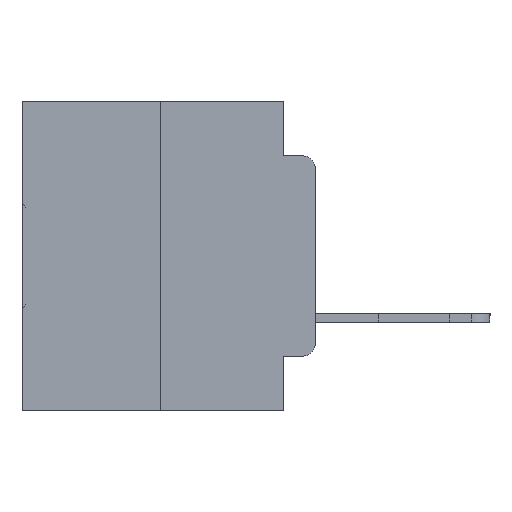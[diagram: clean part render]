
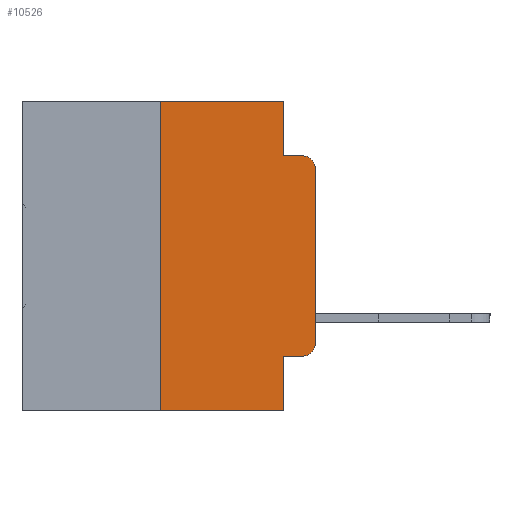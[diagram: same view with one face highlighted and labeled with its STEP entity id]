
A CAD part, left-side view. The second image highlights one B-rep face of the part: STEP entity #10526.
In plain terms, the highlighted planar face has unit normal (-1, 0, 0).
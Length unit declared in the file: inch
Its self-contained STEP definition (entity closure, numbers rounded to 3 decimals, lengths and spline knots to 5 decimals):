
#678 = DIRECTION ( 'NONE',  ( 0., 0., -1. ) ) ;
#717 = DIRECTION ( 'NONE',  ( 0., 0., -1. ) ) ;
#792 = LINE ( 'NONE', #27211, #8308 ) ;
#1229 = DIRECTION ( 'NONE',  ( 0., 0., -1. ) ) ;
#1414 = DIRECTION ( 'NONE',  ( 0., -1., 0. ) ) ;
#2247 = CARTESIAN_POINT ( 'NONE',  ( 0., 0.051, -0.4115 ) ) ;
#2288 = EDGE_CURVE ( 'NONE', #13686, #7421, #14480, .T. ) ;
#2513 = CARTESIAN_POINT ( 'NONE',  ( 0., 0.051, -0.4115 ) ) ;
#2768 = VECTOR ( 'NONE', #20639, 39.37008 ) ;
#4235 = VERTEX_POINT ( 'NONE', #22515 ) ;
#4680 = DIRECTION ( 'NONE',  ( 0., 0., 1. ) ) ;
#5183 = VECTOR ( 'NONE', #1414, 39.37008 ) ;
#5195 = LINE ( 'NONE', #11602, #23070 ) ;
#6860 = EDGE_CURVE ( 'NONE', #8019, #24283, #24549, .T. ) ;
#7421 = VERTEX_POINT ( 'NONE', #30618 ) ;
#7901 = CARTESIAN_POINT ( 'NONE',  ( 0., 0., -0.3915 ) ) ;
#8019 = VERTEX_POINT ( 'NONE', #9274 ) ;
#8308 = VECTOR ( 'NONE', #15422, 39.37008 ) ;
#8387 = VERTEX_POINT ( 'NONE', #8701 ) ;
#8701 = CARTESIAN_POINT ( 'NONE',  ( 0., 0.051, -0.0885 ) ) ;
#8848 = EDGE_CURVE ( 'NONE', #7421, #15583, #22178, .T. ) ;
#9274 = CARTESIAN_POINT ( 'NONE',  ( 0., 0.25, -0.5 ) ) ;
#10526 = ADVANCED_FACE ( 'NONE', ( #15390 ), #11221, .F. ) ;
#10783 = CARTESIAN_POINT ( 'NONE',  ( 0., 0.051, -0.5 ) ) ;
#11136 = LINE ( 'NONE', #28332, #27899 ) ;
#11221 = PLANE ( 'NONE',  #29404 ) ;
#11495 = DIRECTION ( 'NONE',  ( 0., 0., -1. ) ) ;
#11602 = CARTESIAN_POINT ( 'NONE',  ( 0., 0.051, 0. ) ) ;
#11718 = DIRECTION ( 'NONE',  ( 0., -1., 0. ) ) ;
#11909 = DIRECTION ( 'NONE',  ( 0., 0., 1. ) ) ;
#11914 = EDGE_CURVE ( 'NONE', #18131, #8387, #5195, .T. ) ;
#12197 = EDGE_CURVE ( 'NONE', #17667, #24283, #792, .T. ) ;
#13686 = VERTEX_POINT ( 'NONE', #7901 ) ;
#13845 = ORIENTED_EDGE ( 'NONE', *, *, #2288, .T. ) ;
#14002 = CARTESIAN_POINT ( 'NONE',  ( 0., 0.051, 0. ) ) ;
#14480 = LINE ( 'NONE', #18011, #27082 ) ;
#14961 = ORIENTED_EDGE ( 'NONE', *, *, #15974, .F. ) ;
#15008 = DIRECTION ( 'NONE',  ( 0., -1., 0. ) ) ;
#15287 = ORIENTED_EDGE ( 'NONE', *, *, #18986, .F. ) ;
#15313 = AXIS2_PLACEMENT_3D ( 'NONE', #29718, #15635, #717 ) ;
#15390 = FACE_OUTER_BOUND ( 'NONE', #15588, .T. ) ;
#15422 = DIRECTION ( 'NONE',  ( 0., 0., -1. ) ) ;
#15583 = VERTEX_POINT ( 'NONE', #19943 ) ;
#15586 = DIRECTION ( 'NONE',  ( -1., 0., 0. ) ) ;
#15588 = EDGE_LOOP ( 'NONE', ( #13845, #24162, #14961, #22343, #17452, #15287, #20679, #16308, #16558, #19122 ) ) ;
#15635 = DIRECTION ( 'NONE',  ( -1., 0., 0. ) ) ;
#15974 = EDGE_CURVE ( 'NONE', #8387, #15583, #11136, .T. ) ;
#16094 = DIRECTION ( 'NONE',  ( 1., 0., 0. ) ) ;
#16308 = ORIENTED_EDGE ( 'NONE', *, *, #12197, .F. ) ;
#16558 = ORIENTED_EDGE ( 'NONE', *, *, #20662, .T. ) ;
#16653 = CARTESIAN_POINT ( 'NONE',  ( 0., 0.25, 0. ) ) ;
#17452 = ORIENTED_EDGE ( 'NONE', *, *, #26345, .F. ) ;
#17667 = VERTEX_POINT ( 'NONE', #2247 ) ;
#18011 = CARTESIAN_POINT ( 'NONE',  ( 0., 0., 0. ) ) ;
#18090 = LINE ( 'NONE', #16653, #23728 ) ;
#18131 = VERTEX_POINT ( 'NONE', #14002 ) ;
#18177 = CARTESIAN_POINT ( 'NONE',  ( 0., 0.473, 0. ) ) ;
#18642 = CARTESIAN_POINT ( 'NONE',  ( 0., 0.473, -0.5 ) ) ;
#18830 = VERTEX_POINT ( 'NONE', #25703 ) ;
#18986 = EDGE_CURVE ( 'NONE', #8019, #4235, #18090, .T. ) ;
#19122 = ORIENTED_EDGE ( 'NONE', *, *, #28321, .T. ) ;
#19943 = CARTESIAN_POINT ( 'NONE',  ( 0., 0.02, -0.0885 ) ) ;
#20639 = DIRECTION ( 'NONE',  ( 0., -1., 0. ) ) ;
#20662 = EDGE_CURVE ( 'NONE', #17667, #18830, #27985, .T. ) ;
#20679 = ORIENTED_EDGE ( 'NONE', *, *, #6860, .T. ) ;
#21016 = VECTOR ( 'NONE', #15008, 39.37008 ) ;
#22178 = CIRCLE ( 'NONE', #27222, 0.02 ) ;
#22285 = LINE ( 'NONE', #18177, #2768 ) ;
#22343 = ORIENTED_EDGE ( 'NONE', *, *, #11914, .F. ) ;
#22515 = CARTESIAN_POINT ( 'NONE',  ( 0., 0.25, 0. ) ) ;
#23070 = VECTOR ( 'NONE', #11495, 39.37008 ) ;
#23728 = VECTOR ( 'NONE', #11909, 39.37008 ) ;
#24162 = ORIENTED_EDGE ( 'NONE', *, *, #8848, .T. ) ;
#24283 = VERTEX_POINT ( 'NONE', #10783 ) ;
#24549 = LINE ( 'NONE', #18642, #5183 ) ;
#24762 = CIRCLE ( 'NONE', #15313, 0.02 ) ;
#25703 = CARTESIAN_POINT ( 'NONE',  ( 0., 0.02, -0.4115 ) ) ;
#26345 = EDGE_CURVE ( 'NONE', #4235, #18131, #22285, .T. ) ;
#27082 = VECTOR ( 'NONE', #4680, 39.37008 ) ;
#27211 = CARTESIAN_POINT ( 'NONE',  ( 0., 0.051, 0. ) ) ;
#27222 = AXIS2_PLACEMENT_3D ( 'NONE', #29676, #15586, #678 ) ;
#27899 = VECTOR ( 'NONE', #11718, 39.37008 ) ;
#27985 = LINE ( 'NONE', #2513, #21016 ) ;
#28321 = EDGE_CURVE ( 'NONE', #18830, #13686, #24762, .T. ) ;
#28332 = CARTESIAN_POINT ( 'NONE',  ( 0., 0.051, -0.0885 ) ) ;
#29404 = AXIS2_PLACEMENT_3D ( 'NONE', #30088, #16094, #1229 ) ;
#29676 = CARTESIAN_POINT ( 'NONE',  ( 0., 0.02, -0.1085 ) ) ;
#29718 = CARTESIAN_POINT ( 'NONE',  ( 0., 0.02, -0.3915 ) ) ;
#30088 = CARTESIAN_POINT ( 'NONE',  ( 0., 0.473, 0. ) ) ;
#30618 = CARTESIAN_POINT ( 'NONE',  ( 0., 0., -0.1085 ) ) ;
